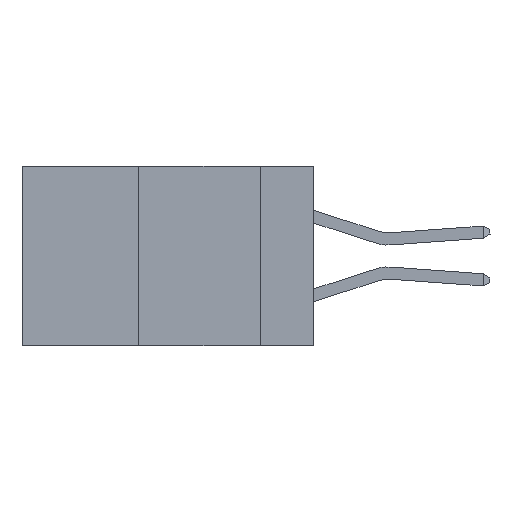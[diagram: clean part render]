
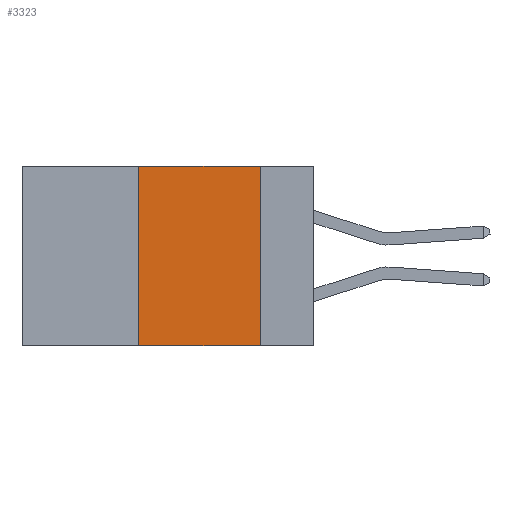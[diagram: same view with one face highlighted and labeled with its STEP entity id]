
A CAD part, left-side view. The second image highlights one B-rep face of the part: STEP entity #3323.
In plain terms, the highlighted planar face has unit normal (-1, 0, 0).
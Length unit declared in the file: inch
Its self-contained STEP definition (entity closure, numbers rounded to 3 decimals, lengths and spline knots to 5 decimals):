
#2 = DIRECTION ( 'NONE',  ( 0., 0., -1. ) ) ;
#15 = VECTOR ( 'NONE', #2, 39.37008 ) ;
#48 = FACE_OUTER_BOUND ( 'NONE', #2187, .T. ) ;
#118 = CARTESIAN_POINT ( 'NONE',  ( 0., 0.6, 0. ) ) ;
#581 = AXIS2_PLACEMENT_3D ( 'NONE', #6208, #5897, #733 ) ;
#641 = VERTEX_POINT ( 'NONE', #8632 ) ;
#733 = DIRECTION ( 'NONE',  ( 0., 0., -1. ) ) ;
#774 = ORIENTED_EDGE ( 'NONE', *, *, #1627, .F. ) ;
#1615 = LINE ( 'NONE', #118, #7649 ) ;
#1627 = EDGE_CURVE ( 'NONE', #3170, #641, #1615, .T. ) ;
#1673 = CARTESIAN_POINT ( 'NONE',  ( 0., 0.36, 0. ) ) ;
#2187 = EDGE_LOOP ( 'NONE', ( #2958, #774, #3065, #4627 ) ) ;
#2911 = LINE ( 'NONE', #3744, #15 ) ;
#2958 = ORIENTED_EDGE ( 'NONE', *, *, #5185, .F. ) ;
#3065 = ORIENTED_EDGE ( 'NONE', *, *, #8343, .F. ) ;
#3142 = VERTEX_POINT ( 'NONE', #3941 ) ;
#3170 = VERTEX_POINT ( 'NONE', #5574 ) ;
#3323 = ADVANCED_FACE ( 'NONE', ( #48 ), #6040, .F. ) ;
#3744 = CARTESIAN_POINT ( 'NONE',  ( 0., 0.11, 0. ) ) ;
#3863 = DIRECTION ( 'NONE',  ( 0., 0., 1. ) ) ;
#3906 = LINE ( 'NONE', #1673, #7901 ) ;
#3941 = CARTESIAN_POINT ( 'NONE',  ( 0., 0.36, -0.37 ) ) ;
#4627 = ORIENTED_EDGE ( 'NONE', *, *, #6808, .T. ) ;
#5185 = EDGE_CURVE ( 'NONE', #641, #6202, #2911, .T. ) ;
#5574 = CARTESIAN_POINT ( 'NONE',  ( 0., 0.36, 0. ) ) ;
#5850 = DIRECTION ( 'NONE',  ( 0., -1., 0. ) ) ;
#5897 = DIRECTION ( 'NONE',  ( 1., 0., 0. ) ) ;
#6040 = PLANE ( 'NONE',  #581 ) ;
#6202 = VERTEX_POINT ( 'NONE', #9276 ) ;
#6208 = CARTESIAN_POINT ( 'NONE',  ( 0., 0.6, 0. ) ) ;
#6808 = EDGE_CURVE ( 'NONE', #3142, #6202, #8581, .T. ) ;
#7441 = VECTOR ( 'NONE', #5850, 39.37008 ) ;
#7649 = VECTOR ( 'NONE', #8946, 39.37008 ) ;
#7901 = VECTOR ( 'NONE', #3863, 39.37008 ) ;
#7961 = CARTESIAN_POINT ( 'NONE',  ( 0., 0.6, -0.37 ) ) ;
#8343 = EDGE_CURVE ( 'NONE', #3142, #3170, #3906, .T. ) ;
#8581 = LINE ( 'NONE', #7961, #7441 ) ;
#8632 = CARTESIAN_POINT ( 'NONE',  ( 0., 0.11, 0. ) ) ;
#8946 = DIRECTION ( 'NONE',  ( 0., -1., 0. ) ) ;
#9276 = CARTESIAN_POINT ( 'NONE',  ( 0., 0.11, -0.37 ) ) ;
